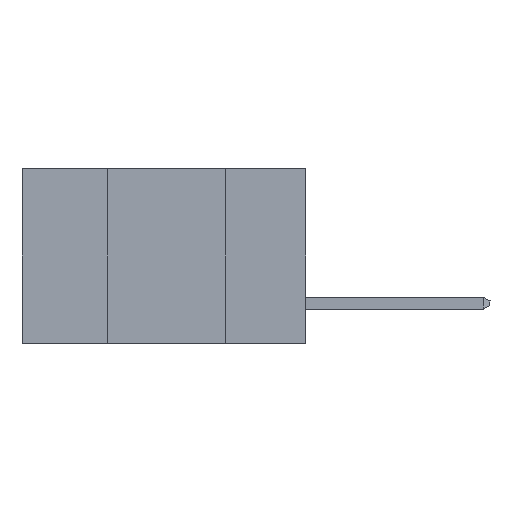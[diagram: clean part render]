
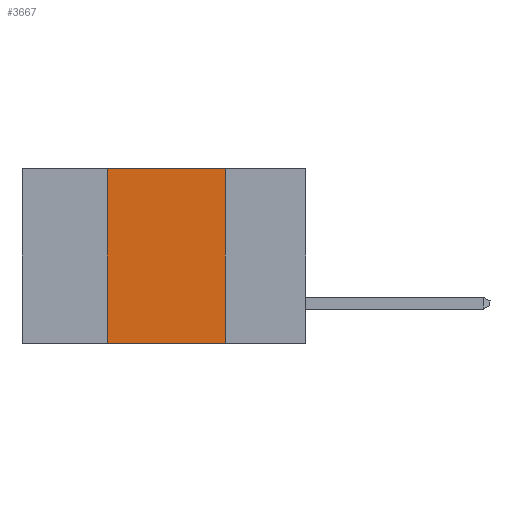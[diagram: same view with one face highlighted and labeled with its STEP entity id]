
A CAD part, left-side view. The second image highlights one B-rep face of the part: STEP entity #3667.
In plain terms, the highlighted planar face has unit normal (-1, 0, 0).
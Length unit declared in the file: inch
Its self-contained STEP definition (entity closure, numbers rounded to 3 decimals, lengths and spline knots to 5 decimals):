
#218 = DIRECTION ( 'NONE',  ( 0., 0., -1. ) ) ;
#1545 = LINE ( 'NONE', #2126, #21344 ) ;
#2126 = CARTESIAN_POINT ( 'NONE',  ( 0., 0.17, 0. ) ) ;
#3249 = EDGE_CURVE ( 'NONE', #11524, #16101, #27000, .T. ) ;
#3667 = ADVANCED_FACE ( 'NONE', ( #23205 ), #13287, .F. ) ;
#3882 = VERTEX_POINT ( 'NONE', #16723 ) ;
#4143 = EDGE_LOOP ( 'NONE', ( #28177, #24543, #6959, #14783 ) ) ;
#6959 = ORIENTED_EDGE ( 'NONE', *, *, #27573, .F. ) ;
#7237 = VERTEX_POINT ( 'NONE', #8189 ) ;
#7487 = AXIS2_PLACEMENT_3D ( 'NONE', #19868, #24467, #218 ) ;
#7512 = CARTESIAN_POINT ( 'NONE',  ( 0., 0.6, -0.37 ) ) ;
#8189 = CARTESIAN_POINT ( 'NONE',  ( 0., 0.17, 0. ) ) ;
#8655 = CARTESIAN_POINT ( 'NONE',  ( 0., 0.42, 0. ) ) ;
#11075 = VECTOR ( 'NONE', #25266, 39.37008 ) ;
#11524 = VERTEX_POINT ( 'NONE', #19435 ) ;
#13287 = PLANE ( 'NONE',  #7487 ) ;
#14783 = ORIENTED_EDGE ( 'NONE', *, *, #3249, .T. ) ;
#15137 = DIRECTION ( 'NONE',  ( 0., 0., 1. ) ) ;
#16101 = VERTEX_POINT ( 'NONE', #17419 ) ;
#16723 = CARTESIAN_POINT ( 'NONE',  ( 0., 0.42, 0. ) ) ;
#17419 = CARTESIAN_POINT ( 'NONE',  ( 0., 0.17, -0.37 ) ) ;
#17557 = LINE ( 'NONE', #24892, #11075 ) ;
#19228 = LINE ( 'NONE', #8655, #21965 ) ;
#19368 = EDGE_CURVE ( 'NONE', #3882, #7237, #17557, .T. ) ;
#19435 = CARTESIAN_POINT ( 'NONE',  ( 0., 0.42, -0.37 ) ) ;
#19829 = VECTOR ( 'NONE', #27231, 39.37008 ) ;
#19868 = CARTESIAN_POINT ( 'NONE',  ( 0., 0.6, 0. ) ) ;
#21344 = VECTOR ( 'NONE', #21980, 39.37008 ) ;
#21965 = VECTOR ( 'NONE', #15137, 39.37008 ) ;
#21980 = DIRECTION ( 'NONE',  ( 0., 0., -1. ) ) ;
#22391 = EDGE_CURVE ( 'NONE', #7237, #16101, #1545, .T. ) ;
#23205 = FACE_OUTER_BOUND ( 'NONE', #4143, .T. ) ;
#24467 = DIRECTION ( 'NONE',  ( 1., 0., 0. ) ) ;
#24543 = ORIENTED_EDGE ( 'NONE', *, *, #19368, .F. ) ;
#24892 = CARTESIAN_POINT ( 'NONE',  ( 0., 0.6, 0. ) ) ;
#25266 = DIRECTION ( 'NONE',  ( 0., -1., 0. ) ) ;
#27000 = LINE ( 'NONE', #7512, #19829 ) ;
#27231 = DIRECTION ( 'NONE',  ( 0., -1., 0. ) ) ;
#27573 = EDGE_CURVE ( 'NONE', #11524, #3882, #19228, .T. ) ;
#28177 = ORIENTED_EDGE ( 'NONE', *, *, #22391, .F. ) ;
